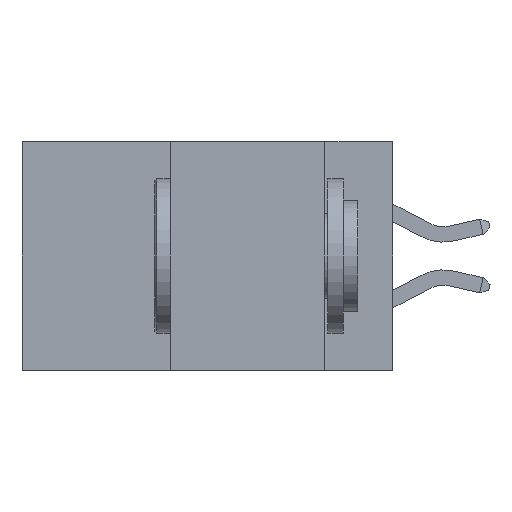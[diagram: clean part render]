
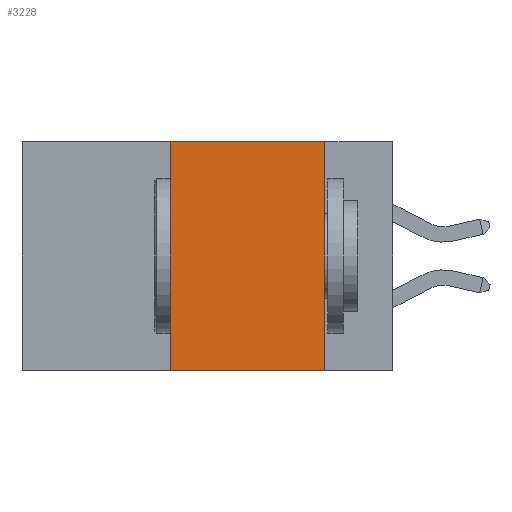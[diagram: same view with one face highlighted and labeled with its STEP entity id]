
A CAD part, left-side view. The second image highlights one B-rep face of the part: STEP entity #3228.
In plain terms, the highlighted planar face has unit normal (-1, 0, 0).
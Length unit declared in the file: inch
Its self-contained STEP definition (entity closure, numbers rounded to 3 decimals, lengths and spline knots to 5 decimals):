
#945 = VERTEX_POINT ( 'NONE', #10489 ) ;
#1411 = LINE ( 'NONE', #3078, #12761 ) ;
#3078 = CARTESIAN_POINT ( 'NONE',  ( 0., 0.6, 0. ) ) ;
#3228 = ADVANCED_FACE ( 'NONE', ( #9129 ), #11492, .F. ) ;
#3410 = LINE ( 'NONE', #14358, #17650 ) ;
#3845 = ORIENTED_EDGE ( 'NONE', *, *, #8410, .T. ) ;
#4938 = CARTESIAN_POINT ( 'NONE',  ( 0., 0.36, 0. ) ) ;
#5023 = EDGE_CURVE ( 'NONE', #14174, #945, #19019, .T. ) ;
#5473 = ORIENTED_EDGE ( 'NONE', *, *, #5023, .F. ) ;
#5544 = DIRECTION ( 'NONE',  ( 0., 0., 1. ) ) ;
#6233 = VERTEX_POINT ( 'NONE', #13312 ) ;
#7096 = DIRECTION ( 'NONE',  ( 0., -1., 0. ) ) ;
#8112 = VERTEX_POINT ( 'NONE', #4938 ) ;
#8410 = EDGE_CURVE ( 'NONE', #6233, #945, #3410, .T. ) ;
#8613 = VECTOR ( 'NONE', #5544, 39.37008 ) ;
#8853 = AXIS2_PLACEMENT_3D ( 'NONE', #17091, #12495, #12475 ) ;
#9024 = DIRECTION ( 'NONE',  ( 0., -1., 0. ) ) ;
#9129 = FACE_OUTER_BOUND ( 'NONE', #13775, .T. ) ;
#10489 = CARTESIAN_POINT ( 'NONE',  ( 0., 0.11, -0.37 ) ) ;
#10821 = ORIENTED_EDGE ( 'NONE', *, *, #18744, .F. ) ;
#10899 = VECTOR ( 'NONE', #18559, 39.37008 ) ;
#11492 = PLANE ( 'NONE',  #8853 ) ;
#12318 = EDGE_CURVE ( 'NONE', #6233, #8112, #16410, .T. ) ;
#12475 = DIRECTION ( 'NONE',  ( 0., 0., -1. ) ) ;
#12495 = DIRECTION ( 'NONE',  ( 1., 0., 0. ) ) ;
#12761 = VECTOR ( 'NONE', #9024, 39.37008 ) ;
#12892 = CARTESIAN_POINT ( 'NONE',  ( 0., 0.36, 0. ) ) ;
#13312 = CARTESIAN_POINT ( 'NONE',  ( 0., 0.36, -0.37 ) ) ;
#13775 = EDGE_LOOP ( 'NONE', ( #5473, #10821, #14685, #3845 ) ) ;
#14174 = VERTEX_POINT ( 'NONE', #16850 ) ;
#14358 = CARTESIAN_POINT ( 'NONE',  ( 0., 0.6, -0.37 ) ) ;
#14685 = ORIENTED_EDGE ( 'NONE', *, *, #12318, .F. ) ;
#16410 = LINE ( 'NONE', #12892, #8613 ) ;
#16686 = CARTESIAN_POINT ( 'NONE',  ( 0., 0.11, 0. ) ) ;
#16850 = CARTESIAN_POINT ( 'NONE',  ( 0., 0.11, 0. ) ) ;
#17091 = CARTESIAN_POINT ( 'NONE',  ( 0., 0.6, 0. ) ) ;
#17650 = VECTOR ( 'NONE', #7096, 39.37008 ) ;
#18559 = DIRECTION ( 'NONE',  ( 0., 0., -1. ) ) ;
#18744 = EDGE_CURVE ( 'NONE', #8112, #14174, #1411, .T. ) ;
#19019 = LINE ( 'NONE', #16686, #10899 ) ;
